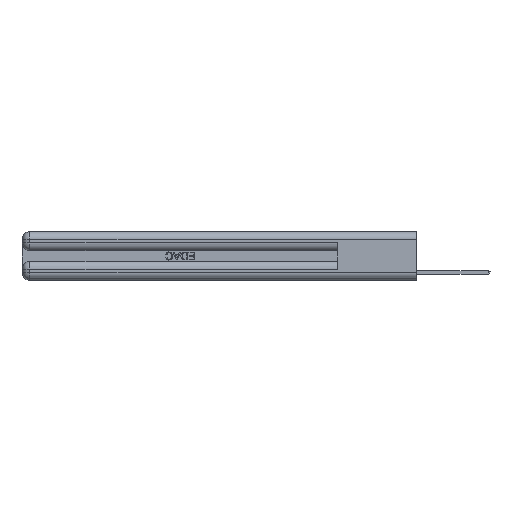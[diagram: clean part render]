
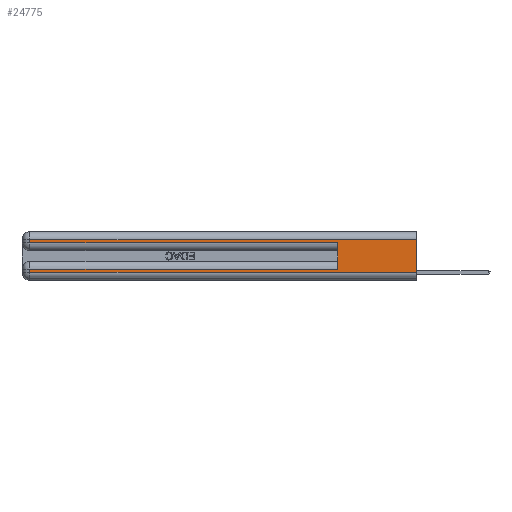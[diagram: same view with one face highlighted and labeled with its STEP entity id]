
A CAD part, left-side view. The second image highlights one B-rep face of the part: STEP entity #24775.
In plain terms, the highlighted planar face has unit normal (-1, 0, 0).
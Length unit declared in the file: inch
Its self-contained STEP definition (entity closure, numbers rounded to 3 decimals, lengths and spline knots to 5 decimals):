
#95 = CARTESIAN_POINT ( 'NONE',  ( 0., 0.6, 0.285 ) ) ;
#460 = DIRECTION ( 'NONE',  ( 0., 1., 0. ) ) ;
#1558 = VERTEX_POINT ( 'NONE', #13726 ) ;
#1590 = EDGE_CURVE ( 'NONE', #1558, #22619, #2735, .T. ) ;
#2735 = LINE ( 'NONE', #24363, #15834 ) ;
#3292 = CARTESIAN_POINT ( 'NONE',  ( 0., 0., 0.37 ) ) ;
#3474 = VERTEX_POINT ( 'NONE', #5013 ) ;
#3508 = LINE ( 'NONE', #25311, #10347 ) ;
#3704 = ORIENTED_EDGE ( 'NONE', *, *, #5728, .F. ) ;
#4349 = VECTOR ( 'NONE', #17210, 39.37008 ) ;
#4380 = CARTESIAN_POINT ( 'NONE',  ( 0., 0., 0.37 ) ) ;
#5013 = CARTESIAN_POINT ( 'NONE',  ( 0., 2.94, 0.085 ) ) ;
#5078 = VECTOR ( 'NONE', #6904, 39.37008 ) ;
#5728 = EDGE_CURVE ( 'NONE', #16221, #32517, #32242, .T. ) ;
#6186 = PLANE ( 'NONE',  #16833 ) ;
#6904 = DIRECTION ( 'NONE',  ( 0., 0., -1. ) ) ;
#7222 = DIRECTION ( 'NONE',  ( 0., 0., 1. ) ) ;
#7549 = LINE ( 'NONE', #26834, #17112 ) ;
#8159 = ORIENTED_EDGE ( 'NONE', *, *, #17255, .F. ) ;
#8298 = DIRECTION ( 'NONE',  ( 0., 1., 0. ) ) ;
#8322 = ORIENTED_EDGE ( 'NONE', *, *, #34046, .T. ) ;
#9404 = ORIENTED_EDGE ( 'NONE', *, *, #24564, .T. ) ;
#10347 = VECTOR ( 'NONE', #460, 39.37008 ) ;
#10677 = DIRECTION ( 'NONE',  ( 0., 0., -1. ) ) ;
#11002 = CARTESIAN_POINT ( 'NONE',  ( 0., 0., 0.085 ) ) ;
#11774 = DIRECTION ( 'NONE',  ( 0., 0., -1. ) ) ;
#13182 = CARTESIAN_POINT ( 'NONE',  ( 0., 0.6, 0.085 ) ) ;
#13726 = CARTESIAN_POINT ( 'NONE',  ( 0., 2.94, 0.31 ) ) ;
#14236 = EDGE_CURVE ( 'NONE', #3474, #25986, #25476, .T. ) ;
#15213 = LINE ( 'NONE', #4380, #5078 ) ;
#15834 = VECTOR ( 'NONE', #10677, 39.37008 ) ;
#16221 = VERTEX_POINT ( 'NONE', #13182 ) ;
#16833 = AXIS2_PLACEMENT_3D ( 'NONE', #3292, #20229, #11774 ) ;
#17112 = VECTOR ( 'NONE', #35452, 39.37008 ) ;
#17210 = DIRECTION ( 'NONE',  ( 0., 0., -1. ) ) ;
#17255 = EDGE_CURVE ( 'NONE', #21392, #34562, #15213, .T. ) ;
#17385 = CARTESIAN_POINT ( 'NONE',  ( 0., 2.94, 0.37 ) ) ;
#18035 = VECTOR ( 'NONE', #29402, 39.37008 ) ;
#18108 = ORIENTED_EDGE ( 'NONE', *, *, #1590, .T. ) ;
#18420 = CARTESIAN_POINT ( 'NONE',  ( 0., 0., 0.285 ) ) ;
#18783 = LINE ( 'NONE', #18420, #18035 ) ;
#19422 = CARTESIAN_POINT ( 'NONE',  ( 0., 0., 0.31 ) ) ;
#19547 = EDGE_LOOP ( 'NONE', ( #8159, #8322, #18108, #9404, #3704, #20664, #34025, #19760 ) ) ;
#19760 = ORIENTED_EDGE ( 'NONE', *, *, #32087, .T. ) ;
#20226 = CARTESIAN_POINT ( 'NONE',  ( 0., 0., 0.06 ) ) ;
#20229 = DIRECTION ( 'NONE',  ( 1., 0., 0. ) ) ;
#20664 = ORIENTED_EDGE ( 'NONE', *, *, #30484, .T. ) ;
#20838 = CARTESIAN_POINT ( 'NONE',  ( 0., 2.94, 0.285 ) ) ;
#21392 = VERTEX_POINT ( 'NONE', #19422 ) ;
#22061 = CARTESIAN_POINT ( 'NONE',  ( 0., 2.94, 0.06 ) ) ;
#22619 = VERTEX_POINT ( 'NONE', #20838 ) ;
#24363 = CARTESIAN_POINT ( 'NONE',  ( 0., 2.94, 0.37 ) ) ;
#24564 = EDGE_CURVE ( 'NONE', #22619, #32517, #18783, .T. ) ;
#24775 = ADVANCED_FACE ( 'NONE', ( #27983 ), #6186, .F. ) ;
#25311 = CARTESIAN_POINT ( 'NONE',  ( 0., 0., 0.31 ) ) ;
#25476 = LINE ( 'NONE', #17385, #4349 ) ;
#25569 = LINE ( 'NONE', #11002, #28611 ) ;
#25986 = VERTEX_POINT ( 'NONE', #22061 ) ;
#26834 = CARTESIAN_POINT ( 'NONE',  ( 0., 0., 0.06 ) ) ;
#27983 = FACE_OUTER_BOUND ( 'NONE', #19547, .T. ) ;
#28611 = VECTOR ( 'NONE', #8298, 39.37008 ) ;
#29402 = DIRECTION ( 'NONE',  ( 0., -1., 0. ) ) ;
#30484 = EDGE_CURVE ( 'NONE', #16221, #3474, #25569, .T. ) ;
#31888 = CARTESIAN_POINT ( 'NONE',  ( 0., 0.6, 0.145 ) ) ;
#32087 = EDGE_CURVE ( 'NONE', #25986, #34562, #7549, .T. ) ;
#32242 = LINE ( 'NONE', #31888, #32348 ) ;
#32348 = VECTOR ( 'NONE', #7222, 39.37008 ) ;
#32517 = VERTEX_POINT ( 'NONE', #95 ) ;
#34025 = ORIENTED_EDGE ( 'NONE', *, *, #14236, .T. ) ;
#34046 = EDGE_CURVE ( 'NONE', #21392, #1558, #3508, .T. ) ;
#34562 = VERTEX_POINT ( 'NONE', #20226 ) ;
#35452 = DIRECTION ( 'NONE',  ( 0., -1., 0. ) ) ;
